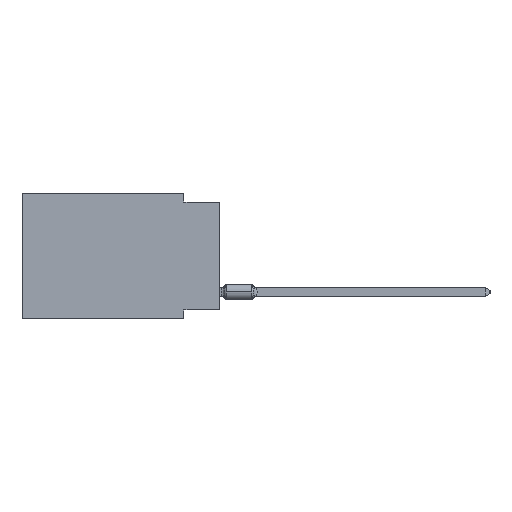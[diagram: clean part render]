
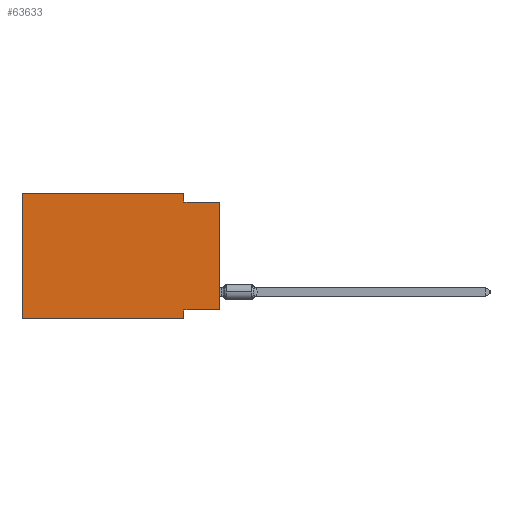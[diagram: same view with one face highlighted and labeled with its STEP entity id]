
A CAD part, left-side view. The second image highlights one B-rep face of the part: STEP entity #63633.
In plain terms, the highlighted planar face has unit normal (-1, 0, 0).
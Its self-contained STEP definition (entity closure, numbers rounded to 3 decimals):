
#1953 = CARTESIAN_POINT ( 'NONE',  ( 0., 13.97, 0. ) ) ;
#4417 = ORIENTED_EDGE ( 'NONE', *, *, #56228, .T. ) ;
#13564 = DIRECTION ( 'NONE',  ( 0., 0., -1. ) ) ;
#16105 = DIRECTION ( 'NONE',  ( 0., 0., -1. ) ) ;
#18235 = FACE_OUTER_BOUND ( 'NONE', #57665, .T. ) ;
#19702 = VERTEX_POINT ( 'NONE', #79519 ) ;
#20501 = VERTEX_POINT ( 'NONE', #42140 ) ;
#20507 = PLANE ( 'NONE',  #58779 ) ;
#24222 = LINE ( 'NONE', #59613, #94041 ) ;
#26165 = LINE ( 'NONE', #103353, #56602 ) ;
#28540 = VECTOR ( 'NONE', #41406, 1000. ) ;
#29410 = DIRECTION ( 'NONE',  ( 0., -1., 0. ) ) ;
#29507 = ORIENTED_EDGE ( 'NONE', *, *, #77055, .F. ) ;
#29569 = CARTESIAN_POINT ( 'NONE',  ( 0., 0., -8.255 ) ) ;
#32196 = VERTEX_POINT ( 'NONE', #65831 ) ;
#35133 = VERTEX_POINT ( 'NONE', #114094 ) ;
#36017 = CARTESIAN_POINT ( 'NONE',  ( 0., 13.97, 0. ) ) ;
#39604 = EDGE_CURVE ( 'NONE', #40758, #19702, #93621, .T. ) ;
#40271 = ORIENTED_EDGE ( 'NONE', *, *, #39604, .F. ) ;
#40758 = VERTEX_POINT ( 'NONE', #36017 ) ;
#40808 = LINE ( 'NONE', #59961, #49388 ) ;
#40832 = CARTESIAN_POINT ( 'NONE',  ( 0., 13.97, 0. ) ) ;
#41406 = DIRECTION ( 'NONE',  ( 0., -1., 0. ) ) ;
#42140 = CARTESIAN_POINT ( 'NONE',  ( 0., 2.54, -8.89 ) ) ;
#44418 = ORIENTED_EDGE ( 'NONE', *, *, #47791, .T. ) ;
#45852 = VERTEX_POINT ( 'NONE', #29569 ) ;
#47350 = EDGE_CURVE ( 'NONE', #32196, #35133, #26165, .T. ) ;
#47791 = EDGE_CURVE ( 'NONE', #45852, #35133, #96341, .T. ) ;
#47871 = ORIENTED_EDGE ( 'NONE', *, *, #48426, .F. ) ;
#48426 = EDGE_CURVE ( 'NONE', #95587, #20501, #40808, .T. ) ;
#49388 = VECTOR ( 'NONE', #13564, 1000. ) ;
#52807 = CARTESIAN_POINT ( 'NONE',  ( 0., 0., 0. ) ) ;
#55525 = LINE ( 'NONE', #92049, #87691 ) ;
#56228 = EDGE_CURVE ( 'NONE', #83322, #20501, #55525, .T. ) ;
#56602 = VECTOR ( 'NONE', #113220, 1000. ) ;
#57665 = EDGE_LOOP ( 'NONE', ( #44418, #71483, #103975, #40271, #65749, #4417, #47871, #29507 ) ) ;
#57714 = LINE ( 'NONE', #94826, #99957 ) ;
#58779 = AXIS2_PLACEMENT_3D ( 'NONE', #1953, #81437, #62922 ) ;
#59613 = CARTESIAN_POINT ( 'NONE',  ( 0., 2.54, 0. ) ) ;
#59961 = CARTESIAN_POINT ( 'NONE',  ( 0., 2.54, -8.89 ) ) ;
#62922 = DIRECTION ( 'NONE',  ( 0., 0., -1. ) ) ;
#63633 = ADVANCED_FACE ( 'NONE', ( #18235 ), #20507, .F. ) ;
#65749 = ORIENTED_EDGE ( 'NONE', *, *, #66733, .F. ) ;
#65831 = CARTESIAN_POINT ( 'NONE',  ( 0., 2.54, -0.635 ) ) ;
#66235 = LINE ( 'NONE', #101023, #74317 ) ;
#66733 = EDGE_CURVE ( 'NONE', #83322, #40758, #57714, .T. ) ;
#71483 = ORIENTED_EDGE ( 'NONE', *, *, #47350, .F. ) ;
#74317 = VECTOR ( 'NONE', #92327, 1000. ) ;
#77055 = EDGE_CURVE ( 'NONE', #45852, #95587, #66235, .T. ) ;
#79519 = CARTESIAN_POINT ( 'NONE',  ( 0., 2.54, 0. ) ) ;
#81437 = DIRECTION ( 'NONE',  ( 1., 0., 0. ) ) ;
#83322 = VERTEX_POINT ( 'NONE', #113835 ) ;
#85116 = EDGE_CURVE ( 'NONE', #19702, #32196, #24222, .T. ) ;
#87691 = VECTOR ( 'NONE', #29410, 1000. ) ;
#88194 = DIRECTION ( 'NONE',  ( 0., 0., 1. ) ) ;
#88249 = VECTOR ( 'NONE', #88194, 1000. ) ;
#92049 = CARTESIAN_POINT ( 'NONE',  ( 0., 13.97, -8.89 ) ) ;
#92327 = DIRECTION ( 'NONE',  ( 0., 1., 0. ) ) ;
#93621 = LINE ( 'NONE', #40832, #28540 ) ;
#93679 = DIRECTION ( 'NONE',  ( 0., 0., 1. ) ) ;
#94041 = VECTOR ( 'NONE', #16105, 1000. ) ;
#94826 = CARTESIAN_POINT ( 'NONE',  ( 0., 13.97, 0. ) ) ;
#95587 = VERTEX_POINT ( 'NONE', #108978 ) ;
#96341 = LINE ( 'NONE', #52807, #88249 ) ;
#99957 = VECTOR ( 'NONE', #93679, 1000. ) ;
#101023 = CARTESIAN_POINT ( 'NONE',  ( 0., 0., -8.255 ) ) ;
#103353 = CARTESIAN_POINT ( 'NONE',  ( 0., 0., -0.635 ) ) ;
#103975 = ORIENTED_EDGE ( 'NONE', *, *, #85116, .F. ) ;
#108978 = CARTESIAN_POINT ( 'NONE',  ( 0., 2.54, -8.255 ) ) ;
#113220 = DIRECTION ( 'NONE',  ( 0., -1., 0. ) ) ;
#113835 = CARTESIAN_POINT ( 'NONE',  ( 0., 13.97, -8.89 ) ) ;
#114094 = CARTESIAN_POINT ( 'NONE',  ( 0., 0., -0.635 ) ) ;
